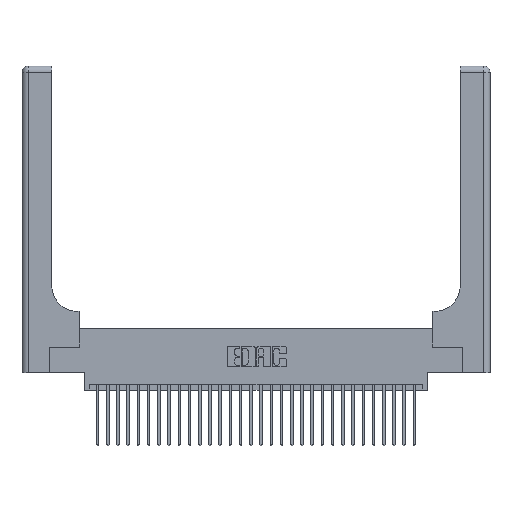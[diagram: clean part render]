
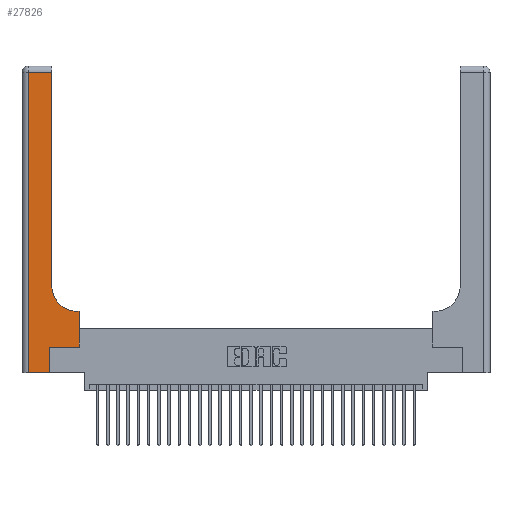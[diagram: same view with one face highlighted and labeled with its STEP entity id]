
A CAD part, top view. The second image highlights one B-rep face of the part: STEP entity #27826.
In plain terms, the highlighted planar face has unit normal (0, 0, 1).
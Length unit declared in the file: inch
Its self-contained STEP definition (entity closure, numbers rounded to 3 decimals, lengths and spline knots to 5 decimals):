
#47 = CARTESIAN_POINT ( 'NONE',  ( 0.5585, 0.25, 0.37 ) ) ;
#647 = DIRECTION ( 'NONE',  ( 0., -1., 0. ) ) ;
#1706 = CARTESIAN_POINT ( 'NONE',  ( 0.2915, 0.6, 0.37 ) ) ;
#1838 = LINE ( 'NONE', #26122, #27944 ) ;
#2346 = ORIENTED_EDGE ( 'NONE', *, *, #9716, .T. ) ;
#2480 = VERTEX_POINT ( 'NONE', #18579 ) ;
#2837 = LINE ( 'NONE', #3388, #17399 ) ;
#2948 = CARTESIAN_POINT ( 'NONE',  ( 0., 3., 0.37 ) ) ;
#3019 = ORIENTED_EDGE ( 'NONE', *, *, #25214, .T. ) ;
#3388 = CARTESIAN_POINT ( 'NONE',  ( 0.2915, 3., 0.37 ) ) ;
#4242 = EDGE_CURVE ( 'NONE', #13126, #29452, #2837, .T. ) ;
#4446 = DIRECTION ( 'NONE',  ( 0., 0., -1. ) ) ;
#5126 = LINE ( 'NONE', #28130, #23925 ) ;
#6749 = ORIENTED_EDGE ( 'NONE', *, *, #24699, .T. ) ;
#6968 = FACE_OUTER_BOUND ( 'NONE', #24153, .T. ) ;
#6981 = DIRECTION ( 'NONE',  ( 1., 0., 0. ) ) ;
#8144 = EDGE_CURVE ( 'NONE', #9869, #13126, #21910, .T. ) ;
#8628 = EDGE_CURVE ( 'NONE', #18844, #24228, #28033, .T. ) ;
#9151 = DIRECTION ( 'NONE',  ( 1., 0., 0. ) ) ;
#9716 = EDGE_CURVE ( 'NONE', #10921, #25479, #1838, .T. ) ;
#9869 = VERTEX_POINT ( 'NONE', #15905 ) ;
#10241 = DIRECTION ( 'NONE',  ( 0., 0., -1. ) ) ;
#10434 = CARTESIAN_POINT ( 'NONE',  ( 0.06, 3., 0.37 ) ) ;
#10544 = VECTOR ( 'NONE', #9151, 39.37008 ) ;
#10885 = VECTOR ( 'NONE', #12526, 39.37008 ) ;
#10921 = VERTEX_POINT ( 'NONE', #14007 ) ;
#11042 = AXIS2_PLACEMENT_3D ( 'NONE', #2948, #10241, #25026 ) ;
#11184 = DIRECTION ( 'NONE',  ( 0., 1., 0. ) ) ;
#11527 = CARTESIAN_POINT ( 'NONE',  ( 0.2915, 0.85, 0.37 ) ) ;
#12526 = DIRECTION ( 'NONE',  ( -1., 0., 0. ) ) ;
#12566 = ORIENTED_EDGE ( 'NONE', *, *, #4242, .T. ) ;
#13126 = VERTEX_POINT ( 'NONE', #11527 ) ;
#14007 = CARTESIAN_POINT ( 'NONE',  ( 0.269, 0., 0.37 ) ) ;
#14590 = LINE ( 'NONE', #47, #27632 ) ;
#15051 = PLANE ( 'NONE',  #11042 ) ;
#15614 = AXIS2_PLACEMENT_3D ( 'NONE', #21567, #4446, #6981 ) ;
#15820 = EDGE_CURVE ( 'NONE', #25479, #2480, #19363, .T. ) ;
#15905 = CARTESIAN_POINT ( 'NONE',  ( 0.5415, 0.6, 0.37 ) ) ;
#17399 = VECTOR ( 'NONE', #11184, 39.37008 ) ;
#18579 = CARTESIAN_POINT ( 'NONE',  ( 0.5585, 0.25, 0.37 ) ) ;
#18844 = VERTEX_POINT ( 'NONE', #19235 ) ;
#18874 = DIRECTION ( 'NONE',  ( -1., 0., 0. ) ) ;
#19222 = CARTESIAN_POINT ( 'NONE',  ( 0.269, 0.25, 0.37 ) ) ;
#19235 = CARTESIAN_POINT ( 'NONE',  ( 0.06, 2.94, 0.37 ) ) ;
#19363 = LINE ( 'NONE', #19222, #10544 ) ;
#19479 = CARTESIAN_POINT ( 'NONE',  ( 0.2915, 2.94, 0.37 ) ) ;
#20923 = ORIENTED_EDGE ( 'NONE', *, *, #22981, .T. ) ;
#21500 = VECTOR ( 'NONE', #647, 39.37008 ) ;
#21567 = CARTESIAN_POINT ( 'NONE',  ( 0.5415, 0.85, 0.37 ) ) ;
#21905 = ORIENTED_EDGE ( 'NONE', *, *, #8144, .T. ) ;
#21910 = CIRCLE ( 'NONE', #15614, 0.25 ) ;
#21978 = ORIENTED_EDGE ( 'NONE', *, *, #8628, .T. ) ;
#22062 = EDGE_CURVE ( 'NONE', #29452, #18844, #27774, .T. ) ;
#22084 = ORIENTED_EDGE ( 'NONE', *, *, #15820, .T. ) ;
#22397 = CARTESIAN_POINT ( 'NONE',  ( 0., 2.94, 0.37 ) ) ;
#22470 = DIRECTION ( 'NONE',  ( 0., 1., 0. ) ) ;
#22658 = VERTEX_POINT ( 'NONE', #31810 ) ;
#22981 = EDGE_CURVE ( 'NONE', #24228, #10921, #5126, .T. ) ;
#23228 = DIRECTION ( 'NONE',  ( 0., 1., 0. ) ) ;
#23925 = VECTOR ( 'NONE', #30360, 39.37008 ) ;
#24153 = EDGE_LOOP ( 'NONE', ( #12566, #30120, #21978, #20923, #2346, #22084, #6749, #3019, #21905 ) ) ;
#24228 = VERTEX_POINT ( 'NONE', #25386 ) ;
#24699 = EDGE_CURVE ( 'NONE', #2480, #22658, #14590, .T. ) ;
#25026 = DIRECTION ( 'NONE',  ( -1., 0., 0. ) ) ;
#25214 = EDGE_CURVE ( 'NONE', #22658, #9869, #31069, .T. ) ;
#25386 = CARTESIAN_POINT ( 'NONE',  ( 0.06, 0., 0.37 ) ) ;
#25479 = VERTEX_POINT ( 'NONE', #27856 ) ;
#26122 = CARTESIAN_POINT ( 'NONE',  ( 0.269, 0., 0.37 ) ) ;
#27632 = VECTOR ( 'NONE', #22470, 39.37008 ) ;
#27774 = LINE ( 'NONE', #22397, #10885 ) ;
#27826 = ADVANCED_FACE ( 'NONE', ( #6968 ), #15051, .F. ) ;
#27856 = CARTESIAN_POINT ( 'NONE',  ( 0.269, 0.25, 0.37 ) ) ;
#27944 = VECTOR ( 'NONE', #23228, 39.37008 ) ;
#28007 = VECTOR ( 'NONE', #18874, 39.37008 ) ;
#28033 = LINE ( 'NONE', #10434, #21500 ) ;
#28130 = CARTESIAN_POINT ( 'NONE',  ( 0., 0., 0.37 ) ) ;
#29452 = VERTEX_POINT ( 'NONE', #19479 ) ;
#30120 = ORIENTED_EDGE ( 'NONE', *, *, #22062, .T. ) ;
#30360 = DIRECTION ( 'NONE',  ( 1., 0., 0. ) ) ;
#31069 = LINE ( 'NONE', #1706, #28007 ) ;
#31810 = CARTESIAN_POINT ( 'NONE',  ( 0.5585, 0.6, 0.37 ) ) ;
